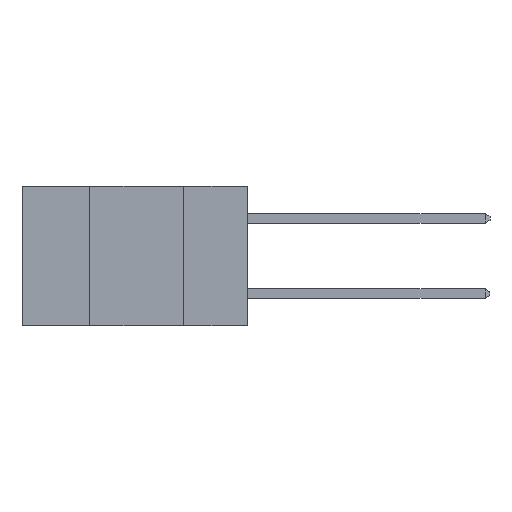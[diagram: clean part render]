
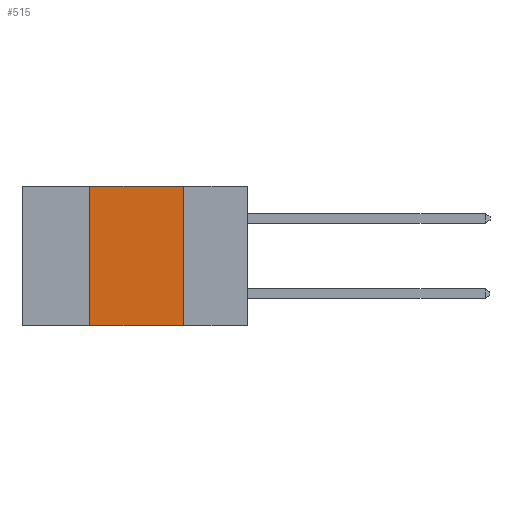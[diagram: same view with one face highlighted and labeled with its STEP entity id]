
A CAD part, left-side view. The second image highlights one B-rep face of the part: STEP entity #515.
In plain terms, the highlighted planar face has unit normal (-1, 0, 0).
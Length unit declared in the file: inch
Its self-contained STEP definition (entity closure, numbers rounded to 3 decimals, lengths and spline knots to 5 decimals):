
#116 = VERTEX_POINT ( 'NONE', #5718 ) ;
#293 = EDGE_CURVE ( 'NONE', #332, #2770, #3907, .T. ) ;
#332 = VERTEX_POINT ( 'NONE', #9191 ) ;
#377 = EDGE_CURVE ( 'NONE', #1039, #116, #8316, .T. ) ;
#515 = ADVANCED_FACE ( 'NONE', ( #9125 ), #3726, .F. ) ;
#1024 = VECTOR ( 'NONE', #3091, 39.37008 ) ;
#1039 = VERTEX_POINT ( 'NONE', #3190 ) ;
#2247 = CARTESIAN_POINT ( 'NONE',  ( 0., 0.6, 0. ) ) ;
#2306 = CARTESIAN_POINT ( 'NONE',  ( 0., 0.6, -0.37 ) ) ;
#2369 = DIRECTION ( 'NONE',  ( 0., -1., 0. ) ) ;
#2770 = VERTEX_POINT ( 'NONE', #10673 ) ;
#2976 = ORIENTED_EDGE ( 'NONE', *, *, #293, .F. ) ;
#3091 = DIRECTION ( 'NONE',  ( 0., 0., 1. ) ) ;
#3190 = CARTESIAN_POINT ( 'NONE',  ( 0., 0.17, 0. ) ) ;
#3726 = PLANE ( 'NONE',  #12346 ) ;
#3907 = LINE ( 'NONE', #4054, #1024 ) ;
#4054 = CARTESIAN_POINT ( 'NONE',  ( 0., 0.42, 0. ) ) ;
#4677 = DIRECTION ( 'NONE',  ( 0., 0., -1. ) ) ;
#4702 = VECTOR ( 'NONE', #9088, 39.37008 ) ;
#5718 = CARTESIAN_POINT ( 'NONE',  ( 0., 0.17, -0.37 ) ) ;
#5772 = EDGE_CURVE ( 'NONE', #2770, #1039, #12735, .T. ) ;
#5990 = DIRECTION ( 'NONE',  ( 0., 0., -1. ) ) ;
#6192 = EDGE_CURVE ( 'NONE', #332, #116, #7636, .T. ) ;
#6829 = VECTOR ( 'NONE', #5990, 39.37008 ) ;
#7636 = LINE ( 'NONE', #2306, #10335 ) ;
#7778 = CARTESIAN_POINT ( 'NONE',  ( 0., 0.17, 0. ) ) ;
#8316 = LINE ( 'NONE', #7778, #6829 ) ;
#9088 = DIRECTION ( 'NONE',  ( 0., -1., 0. ) ) ;
#9125 = FACE_OUTER_BOUND ( 'NONE', #10871, .T. ) ;
#9191 = CARTESIAN_POINT ( 'NONE',  ( 0., 0.42, -0.37 ) ) ;
#10009 = CARTESIAN_POINT ( 'NONE',  ( 0., 0.6, 0. ) ) ;
#10335 = VECTOR ( 'NONE', #2369, 39.37008 ) ;
#10673 = CARTESIAN_POINT ( 'NONE',  ( 0., 0.42, 0. ) ) ;
#10682 = ORIENTED_EDGE ( 'NONE', *, *, #377, .F. ) ;
#10713 = ORIENTED_EDGE ( 'NONE', *, *, #6192, .T. ) ;
#10871 = EDGE_LOOP ( 'NONE', ( #10682, #12626, #2976, #10713 ) ) ;
#12346 = AXIS2_PLACEMENT_3D ( 'NONE', #2247, #13312, #4677 ) ;
#12626 = ORIENTED_EDGE ( 'NONE', *, *, #5772, .F. ) ;
#12735 = LINE ( 'NONE', #10009, #4702 ) ;
#13312 = DIRECTION ( 'NONE',  ( 1., 0., 0. ) ) ;
